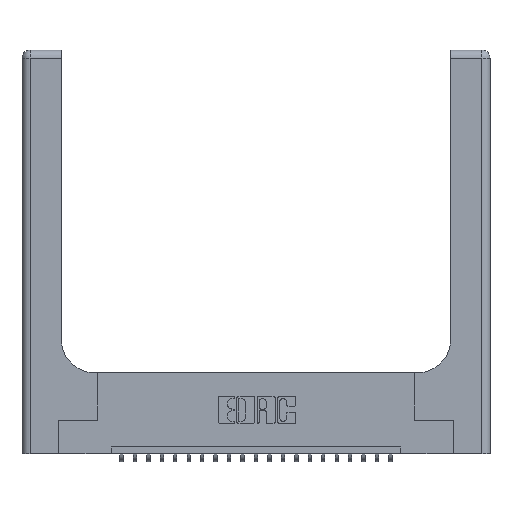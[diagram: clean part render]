
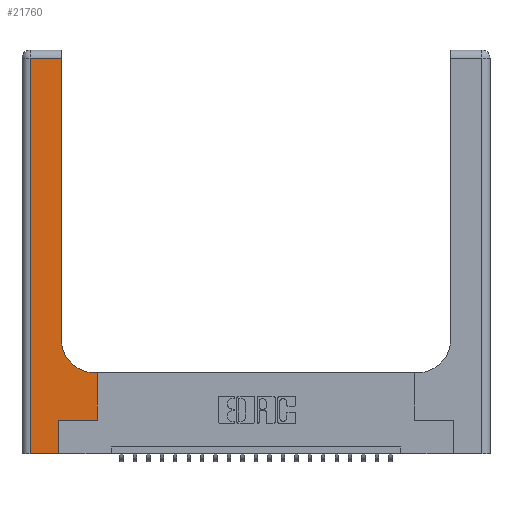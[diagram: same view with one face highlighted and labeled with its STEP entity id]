
A CAD part, top view. The second image highlights one B-rep face of the part: STEP entity #21760.
In plain terms, the highlighted planar face has unit normal (0, 0, 1).
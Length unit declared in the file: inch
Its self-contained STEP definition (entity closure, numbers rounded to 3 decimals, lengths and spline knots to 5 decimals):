
#44 = ORIENTED_EDGE ( 'NONE', *, *, #1219, .T. ) ;
#684 = VERTEX_POINT ( 'NONE', #21603 ) ;
#806 = VERTEX_POINT ( 'NONE', #5400 ) ;
#1030 = CARTESIAN_POINT ( 'NONE',  ( 0.5415, 0.85, 0.37 ) ) ;
#1219 = EDGE_CURVE ( 'NONE', #10330, #17924, #9809, .T. ) ;
#1381 = CARTESIAN_POINT ( 'NONE',  ( 0.06, 3., 0.37 ) ) ;
#1733 = PLANE ( 'NONE',  #18804 ) ;
#3498 = FACE_OUTER_BOUND ( 'NONE', #23374, .T. ) ;
#3629 = CARTESIAN_POINT ( 'NONE',  ( 0.269, 0., 0.37 ) ) ;
#4014 = CARTESIAN_POINT ( 'NONE',  ( 0.2915, 0.6, 0.37 ) ) ;
#4167 = CARTESIAN_POINT ( 'NONE',  ( 0.5585, 0.25, 0.37 ) ) ;
#4590 = VECTOR ( 'NONE', #15223, 39.37008 ) ;
#4662 = LINE ( 'NONE', #4883, #10756 ) ;
#4883 = CARTESIAN_POINT ( 'NONE',  ( 0.269, 0.25, 0.37 ) ) ;
#4920 = VERTEX_POINT ( 'NONE', #10976 ) ;
#5209 = EDGE_CURVE ( 'NONE', #21510, #17110, #17404, .T. ) ;
#5400 = CARTESIAN_POINT ( 'NONE',  ( 0.269, 0.25, 0.37 ) ) ;
#5448 = DIRECTION ( 'NONE',  ( 0., 0., -1. ) ) ;
#5701 = LINE ( 'NONE', #12189, #17830 ) ;
#5850 = CARTESIAN_POINT ( 'NONE',  ( 0.5585, 0.25, 0.37 ) ) ;
#6581 = DIRECTION ( 'NONE',  ( 1., 0., 0. ) ) ;
#6595 = CARTESIAN_POINT ( 'NONE',  ( 0.06, 2.94, 0.37 ) ) ;
#6597 = DIRECTION ( 'NONE',  ( 0., 0., -1. ) ) ;
#6741 = EDGE_CURVE ( 'NONE', #806, #10330, #4662, .T. ) ;
#7033 = CARTESIAN_POINT ( 'NONE',  ( 0.2915, 3., 0.37 ) ) ;
#8488 = AXIS2_PLACEMENT_3D ( 'NONE', #1030, #6597, #15819 ) ;
#9809 = LINE ( 'NONE', #5850, #4590 ) ;
#10330 = VERTEX_POINT ( 'NONE', #4167 ) ;
#10557 = EDGE_CURVE ( 'NONE', #19540, #20095, #10786, .T. ) ;
#10631 = ORIENTED_EDGE ( 'NONE', *, *, #10557, .T. ) ;
#10644 = VECTOR ( 'NONE', #11110, 39.37008 ) ;
#10705 = LINE ( 'NONE', #7033, #19905 ) ;
#10756 = VECTOR ( 'NONE', #6581, 39.37008 ) ;
#10786 = CIRCLE ( 'NONE', #8488, 0.25 ) ;
#10976 = CARTESIAN_POINT ( 'NONE',  ( 0.2915, 2.94, 0.37 ) ) ;
#11110 = DIRECTION ( 'NONE',  ( 0., 1., 0. ) ) ;
#11123 = DIRECTION ( 'NONE',  ( -1., 0., 0. ) ) ;
#11566 = DIRECTION ( 'NONE',  ( -1., 0., 0. ) ) ;
#12189 = CARTESIAN_POINT ( 'NONE',  ( 0., 2.94, 0.37 ) ) ;
#12580 = ORIENTED_EDGE ( 'NONE', *, *, #20616, .T. ) ;
#12848 = LINE ( 'NONE', #14022, #20032 ) ;
#13081 = ORIENTED_EDGE ( 'NONE', *, *, #13412, .T. ) ;
#13168 = CARTESIAN_POINT ( 'NONE',  ( 0.06, 0., 0.37 ) ) ;
#13412 = EDGE_CURVE ( 'NONE', #4920, #21510, #5701, .T. ) ;
#13493 = CARTESIAN_POINT ( 'NONE',  ( 0.5415, 0.6, 0.37 ) ) ;
#13817 = LINE ( 'NONE', #3629, #10644 ) ;
#14022 = CARTESIAN_POINT ( 'NONE',  ( 0., 0., 0.37 ) ) ;
#14521 = CARTESIAN_POINT ( 'NONE',  ( 0.5585, 0.6, 0.37 ) ) ;
#14707 = CARTESIAN_POINT ( 'NONE',  ( 0.2915, 0.85, 0.37 ) ) ;
#15185 = ORIENTED_EDGE ( 'NONE', *, *, #17391, .T. ) ;
#15223 = DIRECTION ( 'NONE',  ( 0., 1., 0. ) ) ;
#15394 = ORIENTED_EDGE ( 'NONE', *, *, #18782, .T. ) ;
#15819 = DIRECTION ( 'NONE',  ( 1., 0., 0. ) ) ;
#16249 = DIRECTION ( 'NONE',  ( 0., 1., 0. ) ) ;
#17110 = VERTEX_POINT ( 'NONE', #13168 ) ;
#17391 = EDGE_CURVE ( 'NONE', #20095, #4920, #10705, .T. ) ;
#17404 = LINE ( 'NONE', #1381, #23438 ) ;
#17791 = DIRECTION ( 'NONE',  ( 1., 0., 0. ) ) ;
#17830 = VECTOR ( 'NONE', #21189, 39.37008 ) ;
#17859 = LINE ( 'NONE', #4014, #20742 ) ;
#17924 = VERTEX_POINT ( 'NONE', #14521 ) ;
#18118 = CARTESIAN_POINT ( 'NONE',  ( 0., 3., 0.37 ) ) ;
#18782 = EDGE_CURVE ( 'NONE', #684, #806, #13817, .T. ) ;
#18804 = AXIS2_PLACEMENT_3D ( 'NONE', #18118, #5448, #11123 ) ;
#19356 = DIRECTION ( 'NONE',  ( 0., -1., 0. ) ) ;
#19540 = VERTEX_POINT ( 'NONE', #13493 ) ;
#19905 = VECTOR ( 'NONE', #16249, 39.37008 ) ;
#20032 = VECTOR ( 'NONE', #17791, 39.37008 ) ;
#20095 = VERTEX_POINT ( 'NONE', #14707 ) ;
#20616 = EDGE_CURVE ( 'NONE', #17110, #684, #12848, .T. ) ;
#20742 = VECTOR ( 'NONE', #11566, 39.37008 ) ;
#20799 = ORIENTED_EDGE ( 'NONE', *, *, #23543, .T. ) ;
#21189 = DIRECTION ( 'NONE',  ( -1., 0., 0. ) ) ;
#21510 = VERTEX_POINT ( 'NONE', #6595 ) ;
#21603 = CARTESIAN_POINT ( 'NONE',  ( 0.269, 0., 0.37 ) ) ;
#21760 = ADVANCED_FACE ( 'NONE', ( #3498 ), #1733, .F. ) ;
#21867 = ORIENTED_EDGE ( 'NONE', *, *, #6741, .T. ) ;
#23374 = EDGE_LOOP ( 'NONE', ( #15185, #13081, #23835, #12580, #15394, #21867, #44, #20799, #10631 ) ) ;
#23438 = VECTOR ( 'NONE', #19356, 39.37008 ) ;
#23543 = EDGE_CURVE ( 'NONE', #17924, #19540, #17859, .T. ) ;
#23835 = ORIENTED_EDGE ( 'NONE', *, *, #5209, .T. ) ;
